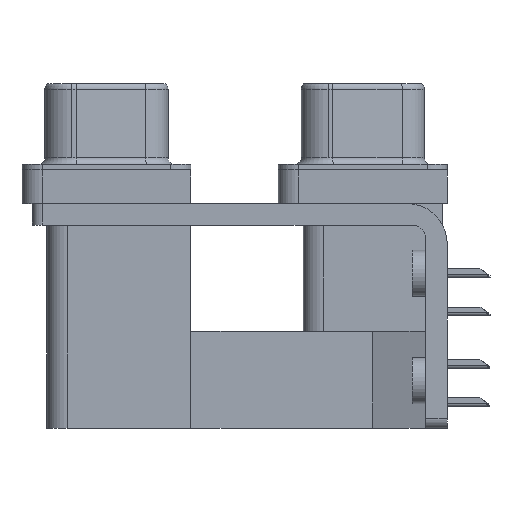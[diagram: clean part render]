
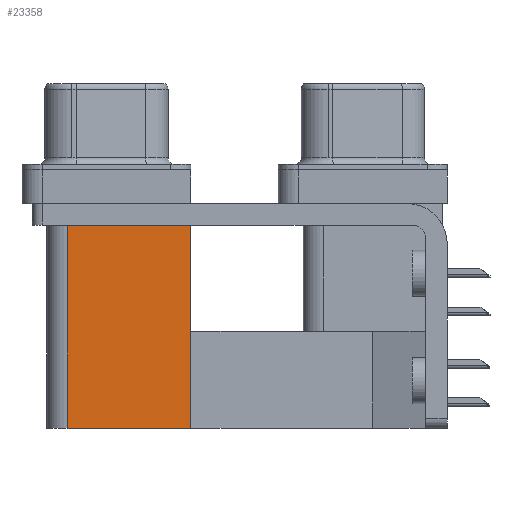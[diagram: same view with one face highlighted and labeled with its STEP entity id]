
A CAD part, left-side view. The second image highlights one B-rep face of the part: STEP entity #23358.
In plain terms, the highlighted planar face has unit normal (-1, 0, 0).
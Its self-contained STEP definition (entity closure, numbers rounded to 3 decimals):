
#194 = ORIENTED_EDGE ( 'NONE', *, *, #25591, .F. ) ;
#325 = EDGE_CURVE ( 'NONE', #10551, #19902, #25339, .T. ) ;
#1289 = EDGE_CURVE ( 'NONE', #24809, #10460, #11482, .T. ) ;
#1606 = VECTOR ( 'NONE', #3439, 1000. ) ;
#3172 = FACE_OUTER_BOUND ( 'NONE', #10071, .T. ) ;
#3435 = CARTESIAN_POINT ( 'NONE',  ( 3.79, 12.775, -2.5 ) ) ;
#3439 = DIRECTION ( 'NONE',  ( 0., 1., 0. ) ) ;
#4318 = ORIENTED_EDGE ( 'NONE', *, *, #325, .F. ) ;
#5239 = PLANE ( 'NONE',  #5781 ) ;
#5365 = CARTESIAN_POINT ( 'NONE',  ( 3.79, 12.775, -19.2 ) ) ;
#5781 = AXIS2_PLACEMENT_3D ( 'NONE', #13195, #12939, #19214 ) ;
#6436 = EDGE_CURVE ( 'NONE', #10551, #24809, #11929, .T. ) ;
#6697 = CARTESIAN_POINT ( 'NONE',  ( 3.79, 21.975, -19.2 ) ) ;
#10071 = EDGE_LOOP ( 'NONE', ( #13725, #194, #4318, #17492 ) ) ;
#10460 = VERTEX_POINT ( 'NONE', #18716 ) ;
#10551 = VERTEX_POINT ( 'NONE', #14676 ) ;
#10818 = VECTOR ( 'NONE', #14514, 1000. ) ;
#11314 = CARTESIAN_POINT ( 'NONE',  ( 3.79, 12.775, -2.5 ) ) ;
#11482 = LINE ( 'NONE', #3435, #25686 ) ;
#11929 = LINE ( 'NONE', #17816, #25335 ) ;
#12939 = DIRECTION ( 'NONE',  ( 1., 0., 0. ) ) ;
#13195 = CARTESIAN_POINT ( 'NONE',  ( 3.79, 12.775, -19.2 ) ) ;
#13725 = ORIENTED_EDGE ( 'NONE', *, *, #1289, .T. ) ;
#14514 = DIRECTION ( 'NONE',  ( 0., 0., 1. ) ) ;
#14676 = CARTESIAN_POINT ( 'NONE',  ( 3.79, 12.775, -19.2 ) ) ;
#17492 = ORIENTED_EDGE ( 'NONE', *, *, #6436, .T. ) ;
#17816 = CARTESIAN_POINT ( 'NONE',  ( 3.79, 12.775, -19.2 ) ) ;
#18716 = CARTESIAN_POINT ( 'NONE',  ( 3.79, 21.975, -2.5 ) ) ;
#19214 = DIRECTION ( 'NONE',  ( 0., 0., -1. ) ) ;
#19902 = VERTEX_POINT ( 'NONE', #21225 ) ;
#19906 = DIRECTION ( 'NONE',  ( 0., 0., 1. ) ) ;
#21225 = CARTESIAN_POINT ( 'NONE',  ( 3.79, 21.975, -19.2 ) ) ;
#23358 = ADVANCED_FACE ( 'NONE', ( #3172 ), #5239, .F. ) ;
#24445 = LINE ( 'NONE', #6697, #10818 ) ;
#24809 = VERTEX_POINT ( 'NONE', #11314 ) ;
#24945 = DIRECTION ( 'NONE',  ( 0., 1., 0. ) ) ;
#25335 = VECTOR ( 'NONE', #19906, 1000. ) ;
#25339 = LINE ( 'NONE', #5365, #1606 ) ;
#25591 = EDGE_CURVE ( 'NONE', #19902, #10460, #24445, .T. ) ;
#25686 = VECTOR ( 'NONE', #24945, 1000. ) ;
